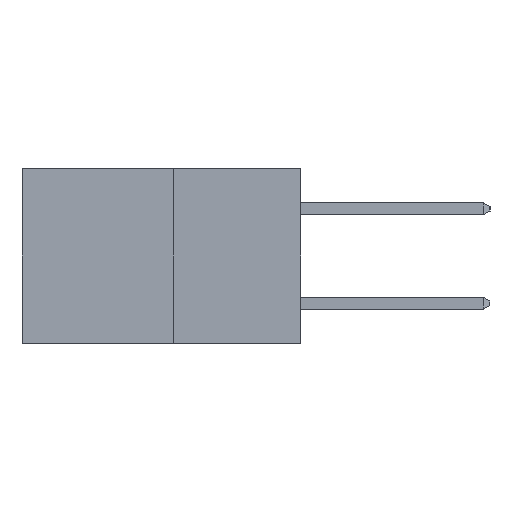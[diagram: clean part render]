
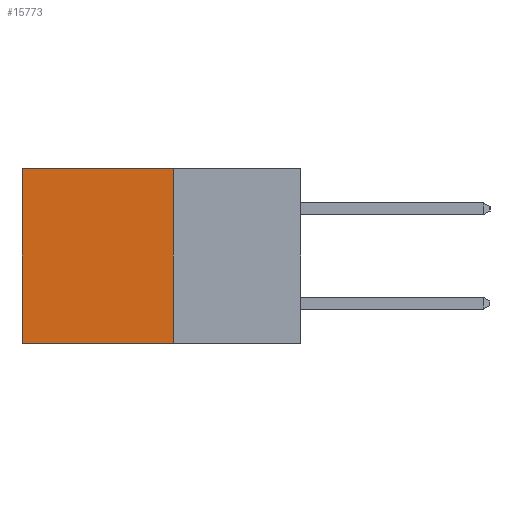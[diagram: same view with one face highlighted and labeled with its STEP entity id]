
A CAD part, left-side view. The second image highlights one B-rep face of the part: STEP entity #15773.
In plain terms, the highlighted planar face has unit normal (-1, 0, 0).
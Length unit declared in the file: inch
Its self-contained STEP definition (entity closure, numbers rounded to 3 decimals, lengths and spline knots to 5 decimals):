
#332 = CARTESIAN_POINT ( 'NONE',  ( 0.277, 0.27, -0.37 ) ) ;
#3263 = LINE ( 'NONE', #9399, #10302 ) ;
#3382 = VERTEX_POINT ( 'NONE', #15131 ) ;
#3642 = AXIS2_PLACEMENT_3D ( 'NONE', #13306, #7040, #15644 ) ;
#3744 = FACE_OUTER_BOUND ( 'NONE', #10418, .T. ) ;
#3826 = EDGE_CURVE ( 'NONE', #8505, #3382, #3263, .T. ) ;
#4037 = DIRECTION ( 'NONE',  ( 0., 0., -1. ) ) ;
#4224 = EDGE_CURVE ( 'NONE', #14936, #11128, #8606, .T. ) ;
#4273 = CARTESIAN_POINT ( 'NONE',  ( 0.277, 0.27, -0.37 ) ) ;
#5168 = VECTOR ( 'NONE', #4037, 39.37008 ) ;
#5629 = VECTOR ( 'NONE', #13895, 39.37008 ) ;
#5785 = PLANE ( 'NONE',  #3642 ) ;
#5987 = CARTESIAN_POINT ( 'NONE',  ( 0.277, 0.27, -0.37 ) ) ;
#6389 = EDGE_CURVE ( 'NONE', #14936, #8505, #9067, .T. ) ;
#7040 = DIRECTION ( 'NONE',  ( 1., 0., 0. ) ) ;
#7673 = CARTESIAN_POINT ( 'NONE',  ( 0.277, 0.27, 0. ) ) ;
#8505 = VERTEX_POINT ( 'NONE', #15023 ) ;
#8606 = LINE ( 'NONE', #4273, #5168 ) ;
#9067 = LINE ( 'NONE', #7673, #5629 ) ;
#9258 = ORIENTED_EDGE ( 'NONE', *, *, #6389, .T. ) ;
#9284 = DIRECTION ( 'NONE',  ( 0., 0., -1. ) ) ;
#9347 = ORIENTED_EDGE ( 'NONE', *, *, #4224, .F. ) ;
#9399 = CARTESIAN_POINT ( 'NONE',  ( 0.277, 0.59, -0.37 ) ) ;
#9565 = ORIENTED_EDGE ( 'NONE', *, *, #10695, .F. ) ;
#9584 = ORIENTED_EDGE ( 'NONE', *, *, #3826, .T. ) ;
#9784 = VECTOR ( 'NONE', #9856, 39.37008 ) ;
#9856 = DIRECTION ( 'NONE',  ( 0., 1., 0. ) ) ;
#10302 = VECTOR ( 'NONE', #9284, 39.37008 ) ;
#10418 = EDGE_LOOP ( 'NONE', ( #9584, #9565, #9347, #9258 ) ) ;
#10695 = EDGE_CURVE ( 'NONE', #11128, #3382, #14114, .T. ) ;
#11128 = VERTEX_POINT ( 'NONE', #332 ) ;
#13306 = CARTESIAN_POINT ( 'NONE',  ( 0.277, 0.27, -0.37 ) ) ;
#13895 = DIRECTION ( 'NONE',  ( 0., 1., 0. ) ) ;
#14114 = LINE ( 'NONE', #5987, #9784 ) ;
#14936 = VERTEX_POINT ( 'NONE', #15706 ) ;
#15023 = CARTESIAN_POINT ( 'NONE',  ( 0.277, 0.59, 0. ) ) ;
#15131 = CARTESIAN_POINT ( 'NONE',  ( 0.277, 0.59, -0.37 ) ) ;
#15644 = DIRECTION ( 'NONE',  ( 0., 0., -1. ) ) ;
#15706 = CARTESIAN_POINT ( 'NONE',  ( 0.277, 0.27, 0. ) ) ;
#15773 = ADVANCED_FACE ( 'NONE', ( #3744 ), #5785, .F. ) ;
